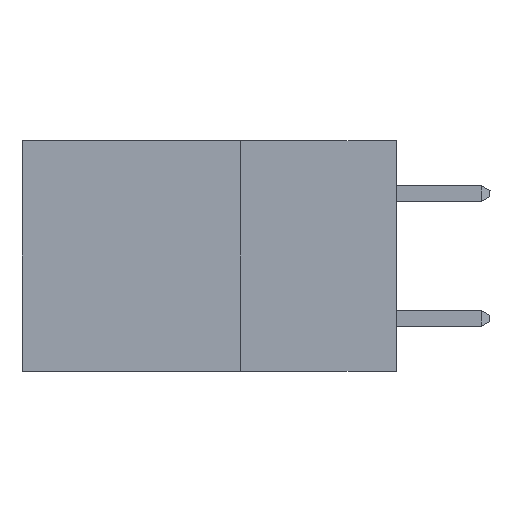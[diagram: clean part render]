
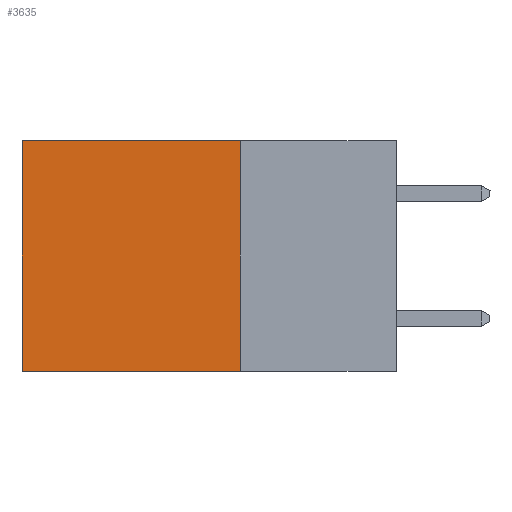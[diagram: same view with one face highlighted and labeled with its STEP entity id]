
A CAD part, left-side view. The second image highlights one B-rep face of the part: STEP entity #3635.
In plain terms, the highlighted planar face has unit normal (-1, 0, 0).
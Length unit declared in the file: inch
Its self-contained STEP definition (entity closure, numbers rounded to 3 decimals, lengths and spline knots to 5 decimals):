
#572 = DIRECTION ( 'NONE',  ( 1., 0., 0. ) ) ;
#850 = CARTESIAN_POINT ( 'NONE',  ( 0.298, 0.25, 0. ) ) ;
#863 = CARTESIAN_POINT ( 'NONE',  ( 0.298, 0.25, 0. ) ) ;
#895 = PLANE ( 'NONE',  #18856 ) ;
#1999 = VERTEX_POINT ( 'NONE', #27796 ) ;
#2194 = CARTESIAN_POINT ( 'NONE',  ( 0.298, 0.25, -0.37 ) ) ;
#2310 = LINE ( 'NONE', #24800, #19401 ) ;
#2562 = ORIENTED_EDGE ( 'NONE', *, *, #22724, .T. ) ;
#2594 = DIRECTION ( 'NONE',  ( 0., 0., -1. ) ) ;
#3196 = CARTESIAN_POINT ( 'NONE',  ( 0.298, 0.25, 0. ) ) ;
#3635 = ADVANCED_FACE ( 'NONE', ( #27051 ), #895, .F. ) ;
#4216 = EDGE_LOOP ( 'NONE', ( #2562, #18935, #7713, #15470 ) ) ;
#4991 = LINE ( 'NONE', #2194, #20602 ) ;
#6718 = EDGE_CURVE ( 'NONE', #12218, #7129, #4991, .T. ) ;
#7129 = VERTEX_POINT ( 'NONE', #25564 ) ;
#7167 = DIRECTION ( 'NONE',  ( 0., 1., 0. ) ) ;
#7713 = ORIENTED_EDGE ( 'NONE', *, *, #24222, .F. ) ;
#9651 = LINE ( 'NONE', #850, #16236 ) ;
#9836 = EDGE_CURVE ( 'NONE', #18761, #1999, #2310, .T. ) ;
#10247 = CARTESIAN_POINT ( 'NONE',  ( 0.298, 0.25, -0.37 ) ) ;
#11295 = DIRECTION ( 'NONE',  ( 0., 1., 0. ) ) ;
#12218 = VERTEX_POINT ( 'NONE', #10247 ) ;
#15470 = ORIENTED_EDGE ( 'NONE', *, *, #9836, .T. ) ;
#15728 = DIRECTION ( 'NONE',  ( 0., 0., -1. ) ) ;
#16001 = CARTESIAN_POINT ( 'NONE',  ( 0.298, 0.6, 0. ) ) ;
#16236 = VECTOR ( 'NONE', #23160, 39.37008 ) ;
#18761 = VERTEX_POINT ( 'NONE', #3196 ) ;
#18856 = AXIS2_PLACEMENT_3D ( 'NONE', #863, #572, #15728 ) ;
#18935 = ORIENTED_EDGE ( 'NONE', *, *, #6718, .F. ) ;
#19401 = VECTOR ( 'NONE', #7167, 39.37008 ) ;
#20602 = VECTOR ( 'NONE', #11295, 39.37008 ) ;
#21841 = VECTOR ( 'NONE', #2594, 39.37008 ) ;
#22724 = EDGE_CURVE ( 'NONE', #1999, #7129, #26894, .T. ) ;
#23160 = DIRECTION ( 'NONE',  ( 0., 0., -1. ) ) ;
#24222 = EDGE_CURVE ( 'NONE', #18761, #12218, #9651, .T. ) ;
#24800 = CARTESIAN_POINT ( 'NONE',  ( 0.298, 0.25, 0. ) ) ;
#25564 = CARTESIAN_POINT ( 'NONE',  ( 0.298, 0.6, -0.37 ) ) ;
#26894 = LINE ( 'NONE', #16001, #21841 ) ;
#27051 = FACE_OUTER_BOUND ( 'NONE', #4216, .T. ) ;
#27796 = CARTESIAN_POINT ( 'NONE',  ( 0.298, 0.6, 0. ) ) ;
